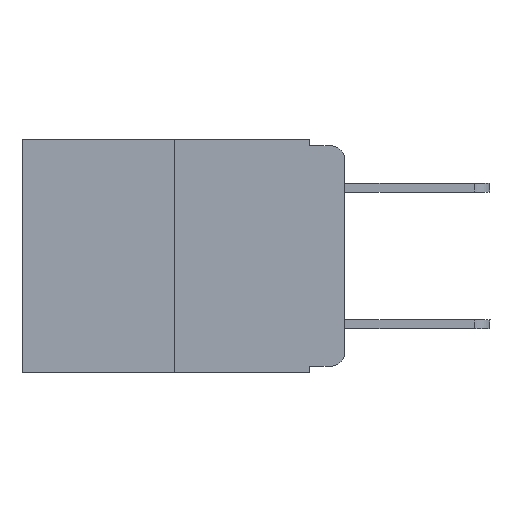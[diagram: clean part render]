
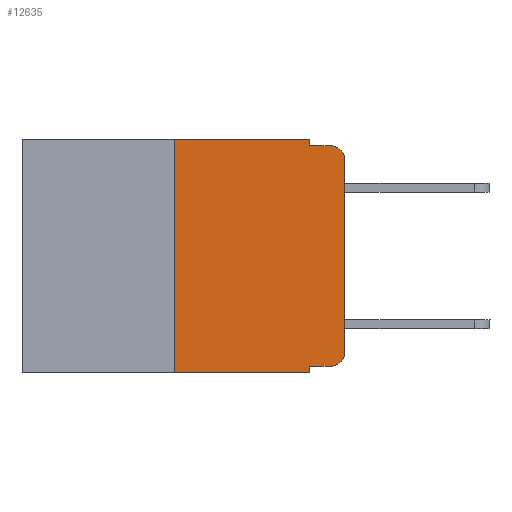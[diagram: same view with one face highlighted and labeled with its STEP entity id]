
A CAD part, left-side view. The second image highlights one B-rep face of the part: STEP entity #12635.
In plain terms, the highlighted planar face has unit normal (-1, 0, 0).
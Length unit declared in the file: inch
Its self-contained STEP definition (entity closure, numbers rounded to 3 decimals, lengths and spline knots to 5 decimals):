
#139 = DIRECTION ( 'NONE',  ( 0., 0., -1. ) ) ;
#204 = VECTOR ( 'NONE', #19006, 39.37008 ) ;
#358 = LINE ( 'NONE', #4296, #7939 ) ;
#390 = LINE ( 'NONE', #7879, #575 ) ;
#575 = VECTOR ( 'NONE', #139, 39.37008 ) ;
#775 = DIRECTION ( 'NONE',  ( 0., 0., -1. ) ) ;
#1356 = VERTEX_POINT ( 'NONE', #3294 ) ;
#1616 = CARTESIAN_POINT ( 'NONE',  ( 0., 0.473, 0. ) ) ;
#1742 = EDGE_CURVE ( 'NONE', #10573, #18997, #14954, .T. ) ;
#1881 = CARTESIAN_POINT ( 'NONE',  ( 0., 0.473, -0.343 ) ) ;
#1973 = LINE ( 'NONE', #1616, #5187 ) ;
#2059 = LINE ( 'NONE', #15395, #21211 ) ;
#2116 = CARTESIAN_POINT ( 'NONE',  ( 0., 0.02, -0.313 ) ) ;
#2480 = CARTESIAN_POINT ( 'NONE',  ( 0., 0.051, -0.01 ) ) ;
#3227 = EDGE_CURVE ( 'NONE', #18997, #21293, #13997, .T. ) ;
#3294 = CARTESIAN_POINT ( 'NONE',  ( 0., 0.051, 0. ) ) ;
#3659 = CARTESIAN_POINT ( 'NONE',  ( 0., 0.473, 0. ) ) ;
#4296 = CARTESIAN_POINT ( 'NONE',  ( 0., 0., 0. ) ) ;
#4662 = VECTOR ( 'NONE', #775, 39.37008 ) ;
#4950 = AXIS2_PLACEMENT_3D ( 'NONE', #12704, #10926, #18434 ) ;
#5187 = VECTOR ( 'NONE', #22811, 39.37008 ) ;
#6441 = EDGE_CURVE ( 'NONE', #1356, #22535, #18164, .T. ) ;
#6974 = VECTOR ( 'NONE', #15196, 39.37008 ) ;
#7879 = CARTESIAN_POINT ( 'NONE',  ( 0., 0.051, 0. ) ) ;
#7939 = VECTOR ( 'NONE', #22065, 39.37008 ) ;
#8261 = CARTESIAN_POINT ( 'NONE',  ( 0., 0., -0.03 ) ) ;
#8554 = VERTEX_POINT ( 'NONE', #10009 ) ;
#8555 = CARTESIAN_POINT ( 'NONE',  ( 0., 0.25, 0. ) ) ;
#8976 = CARTESIAN_POINT ( 'NONE',  ( 0., 0.051, -0.333 ) ) ;
#9009 = CIRCLE ( 'NONE', #4950, 0.02 ) ;
#9273 = EDGE_CURVE ( 'NONE', #8554, #1356, #1973, .T. ) ;
#9479 = FACE_OUTER_BOUND ( 'NONE', #10177, .T. ) ;
#9681 = VECTOR ( 'NONE', #16185, 39.37008 ) ;
#9863 = VERTEX_POINT ( 'NONE', #8261 ) ;
#9865 = LINE ( 'NONE', #8555, #9681 ) ;
#10009 = CARTESIAN_POINT ( 'NONE',  ( 0., 0.25, 0. ) ) ;
#10154 = CARTESIAN_POINT ( 'NONE',  ( 0., 0.051, 0. ) ) ;
#10177 = EDGE_LOOP ( 'NONE', ( #22954, #17856, #20660, #11943, #24372, #23784, #10831, #24942, #17589, #16650 ) ) ;
#10573 = VERTEX_POINT ( 'NONE', #21775 ) ;
#10831 = ORIENTED_EDGE ( 'NONE', *, *, #23505, .T. ) ;
#10926 = DIRECTION ( 'NONE',  ( -1., 0., 0. ) ) ;
#11258 = LINE ( 'NONE', #1881, #204 ) ;
#11940 = EDGE_CURVE ( 'NONE', #18437, #8554, #9865, .T. ) ;
#11943 = ORIENTED_EDGE ( 'NONE', *, *, #6441, .F. ) ;
#12635 = ADVANCED_FACE ( 'NONE', ( #9479 ), #17490, .F. ) ;
#12704 = CARTESIAN_POINT ( 'NONE',  ( 0., 0.02, -0.03 ) ) ;
#13997 = CIRCLE ( 'NONE', #21306, 0.02 ) ;
#14485 = CARTESIAN_POINT ( 'NONE',  ( 0., 0.02, -0.01 ) ) ;
#14954 = LINE ( 'NONE', #8976, #6974 ) ;
#15190 = EDGE_CURVE ( 'NONE', #9863, #21620, #9009, .T. ) ;
#15196 = DIRECTION ( 'NONE',  ( 0., -1., 0. ) ) ;
#15395 = CARTESIAN_POINT ( 'NONE',  ( 0., 0.051, -0.01 ) ) ;
#15397 = AXIS2_PLACEMENT_3D ( 'NONE', #3659, #17115, #15594 ) ;
#15594 = DIRECTION ( 'NONE',  ( 0., 0., -1. ) ) ;
#16185 = DIRECTION ( 'NONE',  ( 0., 0., 1. ) ) ;
#16577 = CARTESIAN_POINT ( 'NONE',  ( 0., 0.25, -0.343 ) ) ;
#16650 = ORIENTED_EDGE ( 'NONE', *, *, #3227, .T. ) ;
#16923 = CARTESIAN_POINT ( 'NONE',  ( 0., 0.02, -0.333 ) ) ;
#17115 = DIRECTION ( 'NONE',  ( 1., 0., 0. ) ) ;
#17301 = CARTESIAN_POINT ( 'NONE',  ( 0., 0.051, -0.343 ) ) ;
#17360 = DIRECTION ( 'NONE',  ( -1., 0., 0. ) ) ;
#17490 = PLANE ( 'NONE',  #15397 ) ;
#17589 = ORIENTED_EDGE ( 'NONE', *, *, #1742, .T. ) ;
#17731 = EDGE_CURVE ( 'NONE', #21293, #9863, #358, .T. ) ;
#17856 = ORIENTED_EDGE ( 'NONE', *, *, #15190, .T. ) ;
#18164 = LINE ( 'NONE', #10154, #4662 ) ;
#18434 = DIRECTION ( 'NONE',  ( 0., 0., -1. ) ) ;
#18437 = VERTEX_POINT ( 'NONE', #16577 ) ;
#18997 = VERTEX_POINT ( 'NONE', #16923 ) ;
#19006 = DIRECTION ( 'NONE',  ( 0., -1., 0. ) ) ;
#20290 = EDGE_CURVE ( 'NONE', #22535, #21620, #2059, .T. ) ;
#20660 = ORIENTED_EDGE ( 'NONE', *, *, #20290, .F. ) ;
#21211 = VECTOR ( 'NONE', #21224, 39.37008 ) ;
#21224 = DIRECTION ( 'NONE',  ( 0., -1., 0. ) ) ;
#21293 = VERTEX_POINT ( 'NONE', #24146 ) ;
#21306 = AXIS2_PLACEMENT_3D ( 'NONE', #2116, #17360, #21662 ) ;
#21620 = VERTEX_POINT ( 'NONE', #14485 ) ;
#21662 = DIRECTION ( 'NONE',  ( 0., 0., -1. ) ) ;
#21775 = CARTESIAN_POINT ( 'NONE',  ( 0., 0.051, -0.333 ) ) ;
#22065 = DIRECTION ( 'NONE',  ( 0., 0., 1. ) ) ;
#22535 = VERTEX_POINT ( 'NONE', #2480 ) ;
#22796 = EDGE_CURVE ( 'NONE', #10573, #24456, #390, .T. ) ;
#22811 = DIRECTION ( 'NONE',  ( 0., -1., 0. ) ) ;
#22954 = ORIENTED_EDGE ( 'NONE', *, *, #17731, .T. ) ;
#23505 = EDGE_CURVE ( 'NONE', #18437, #24456, #11258, .T. ) ;
#23784 = ORIENTED_EDGE ( 'NONE', *, *, #11940, .F. ) ;
#24146 = CARTESIAN_POINT ( 'NONE',  ( 0., 0., -0.313 ) ) ;
#24372 = ORIENTED_EDGE ( 'NONE', *, *, #9273, .F. ) ;
#24456 = VERTEX_POINT ( 'NONE', #17301 ) ;
#24942 = ORIENTED_EDGE ( 'NONE', *, *, #22796, .F. ) ;
